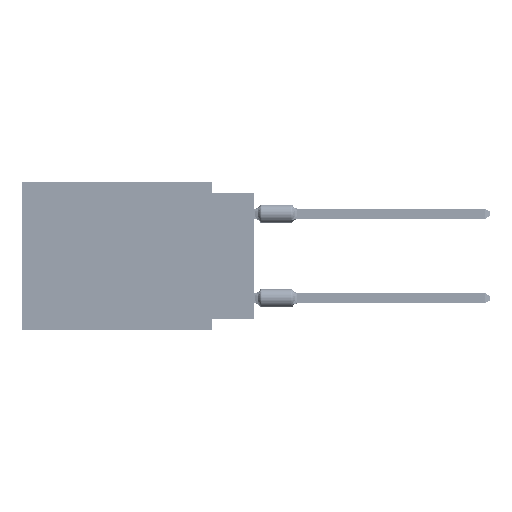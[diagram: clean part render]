
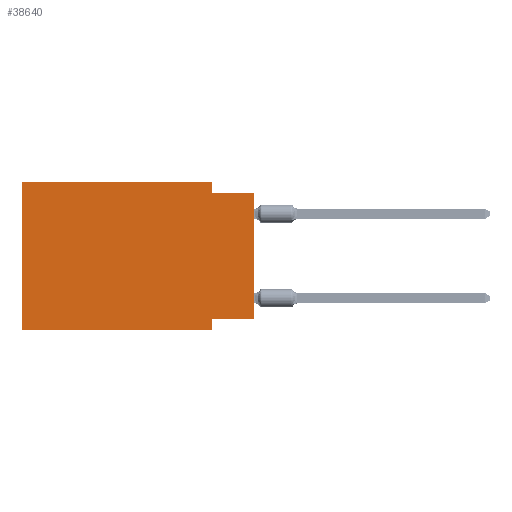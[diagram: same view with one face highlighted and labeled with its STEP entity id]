
A CAD part, left-side view. The second image highlights one B-rep face of the part: STEP entity #38640.
In plain terms, the highlighted planar face has unit normal (-1, 0, 0).
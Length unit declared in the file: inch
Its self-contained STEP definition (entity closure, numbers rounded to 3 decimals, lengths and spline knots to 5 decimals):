
#388 = CARTESIAN_POINT ( 'NONE',  ( 0., 0., -0.025 ) ) ;
#569 = EDGE_CURVE ( 'NONE', #80386, #11169, #37917, .T. ) ;
#586 = CARTESIAN_POINT ( 'NONE',  ( 0., 0.1, -0.35 ) ) ;
#1818 = EDGE_LOOP ( 'NONE', ( #15054, #16562, #38416, #63165, #66525, #42550, #36568, #65613 ) ) ;
#2611 = LINE ( 'NONE', #586, #32721 ) ;
#3765 = VECTOR ( 'NONE', #46385, 39.37008 ) ;
#8009 = CARTESIAN_POINT ( 'NONE',  ( 0., 0., 0. ) ) ;
#8193 = CARTESIAN_POINT ( 'NONE',  ( 0., 0., -0.325 ) ) ;
#8298 = CARTESIAN_POINT ( 'NONE',  ( 0., 0.1, -0.025 ) ) ;
#11169 = VERTEX_POINT ( 'NONE', #57788 ) ;
#12470 = VECTOR ( 'NONE', #50311, 39.37008 ) ;
#14117 = DIRECTION ( 'NONE',  ( 0., 0., -1. ) ) ;
#14804 = VERTEX_POINT ( 'NONE', #8298 ) ;
#15054 = ORIENTED_EDGE ( 'NONE', *, *, #569, .T. ) ;
#16373 = CARTESIAN_POINT ( 'NONE',  ( 0., 0.1, 0. ) ) ;
#16562 = ORIENTED_EDGE ( 'NONE', *, *, #29081, .F. ) ;
#16768 = VECTOR ( 'NONE', #72265, 39.37008 ) ;
#19304 = CARTESIAN_POINT ( 'NONE',  ( 0., 0.55, 0. ) ) ;
#20584 = VECTOR ( 'NONE', #34769, 39.37008 ) ;
#22221 = VERTEX_POINT ( 'NONE', #26044 ) ;
#22575 = CARTESIAN_POINT ( 'NONE',  ( 0., 0.55, -0.35 ) ) ;
#25169 = EDGE_CURVE ( 'NONE', #22221, #71042, #2611, .T. ) ;
#25715 = VERTEX_POINT ( 'NONE', #19304 ) ;
#26044 = CARTESIAN_POINT ( 'NONE',  ( 0., 0.1, -0.325 ) ) ;
#29081 = EDGE_CURVE ( 'NONE', #14804, #11169, #46239, .T. ) ;
#29292 = CARTESIAN_POINT ( 'NONE',  ( 0., 0.1, -0.35 ) ) ;
#31148 = LINE ( 'NONE', #22575, #80152 ) ;
#32721 = VECTOR ( 'NONE', #71128, 39.37008 ) ;
#34769 = DIRECTION ( 'NONE',  ( 0., 0., 1. ) ) ;
#36568 = ORIENTED_EDGE ( 'NONE', *, *, #25169, .F. ) ;
#37917 = LINE ( 'NONE', #8009, #3765 ) ;
#38416 = ORIENTED_EDGE ( 'NONE', *, *, #49153, .F. ) ;
#38640 = ADVANCED_FACE ( 'NONE', ( #82062 ), #46009, .F. ) ;
#39096 = DIRECTION ( 'NONE',  ( 0., -1., 0. ) ) ;
#39253 = CARTESIAN_POINT ( 'NONE',  ( 0., 0.55, 0. ) ) ;
#39374 = CARTESIAN_POINT ( 'NONE',  ( 0., 0.55, 0. ) ) ;
#42550 = ORIENTED_EDGE ( 'NONE', *, *, #76868, .T. ) ;
#45209 = VERTEX_POINT ( 'NONE', #16373 ) ;
#45861 = DIRECTION ( 'NONE',  ( 0., -1., 0. ) ) ;
#46009 = PLANE ( 'NONE',  #74211 ) ;
#46239 = LINE ( 'NONE', #388, #78241 ) ;
#46385 = DIRECTION ( 'NONE',  ( 0., 0., 1. ) ) ;
#49153 = EDGE_CURVE ( 'NONE', #45209, #14804, #63470, .T. ) ;
#49190 = VECTOR ( 'NONE', #45861, 39.37008 ) ;
#50311 = DIRECTION ( 'NONE',  ( 0., 0., -1. ) ) ;
#52388 = DIRECTION ( 'NONE',  ( 1., 0., 0. ) ) ;
#54412 = CARTESIAN_POINT ( 'NONE',  ( 0., 0.55, -0.35 ) ) ;
#57788 = CARTESIAN_POINT ( 'NONE',  ( 0., 0., -0.025 ) ) ;
#62382 = VERTEX_POINT ( 'NONE', #54412 ) ;
#63165 = ORIENTED_EDGE ( 'NONE', *, *, #76618, .F. ) ;
#63470 = LINE ( 'NONE', #82198, #12470 ) ;
#65565 = LINE ( 'NONE', #73045, #20584 ) ;
#65613 = ORIENTED_EDGE ( 'NONE', *, *, #78734, .F. ) ;
#65717 = LINE ( 'NONE', #8193, #16768 ) ;
#66130 = LINE ( 'NONE', #39374, #49190 ) ;
#66525 = ORIENTED_EDGE ( 'NONE', *, *, #82799, .F. ) ;
#67428 = CARTESIAN_POINT ( 'NONE',  ( 0., 0., -0.325 ) ) ;
#71042 = VERTEX_POINT ( 'NONE', #29292 ) ;
#71128 = DIRECTION ( 'NONE',  ( 0., 0., -1. ) ) ;
#72265 = DIRECTION ( 'NONE',  ( 0., 1., 0. ) ) ;
#73045 = CARTESIAN_POINT ( 'NONE',  ( 0., 0.55, 0. ) ) ;
#73735 = DIRECTION ( 'NONE',  ( 0., -1., 0. ) ) ;
#74211 = AXIS2_PLACEMENT_3D ( 'NONE', #39253, #52388, #14117 ) ;
#76618 = EDGE_CURVE ( 'NONE', #25715, #45209, #66130, .T. ) ;
#76868 = EDGE_CURVE ( 'NONE', #62382, #71042, #31148, .T. ) ;
#78241 = VECTOR ( 'NONE', #39096, 39.37008 ) ;
#78734 = EDGE_CURVE ( 'NONE', #80386, #22221, #65717, .T. ) ;
#80152 = VECTOR ( 'NONE', #73735, 39.37008 ) ;
#80386 = VERTEX_POINT ( 'NONE', #67428 ) ;
#82062 = FACE_OUTER_BOUND ( 'NONE', #1818, .T. ) ;
#82198 = CARTESIAN_POINT ( 'NONE',  ( 0., 0.1, 0. ) ) ;
#82799 = EDGE_CURVE ( 'NONE', #62382, #25715, #65565, .T. ) ;
